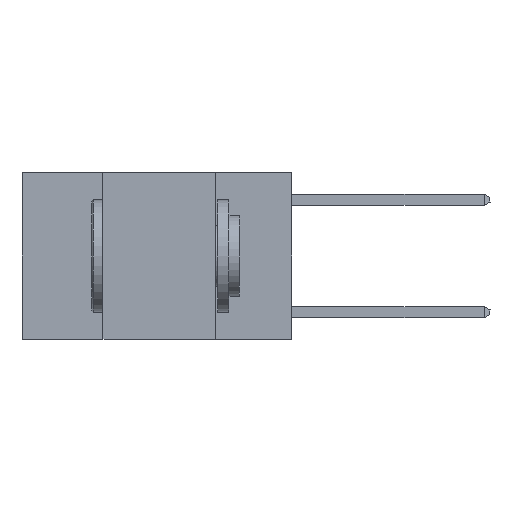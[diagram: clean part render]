
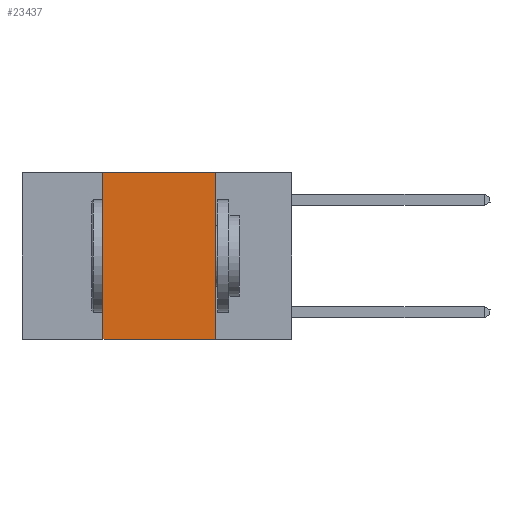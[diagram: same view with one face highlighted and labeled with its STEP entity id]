
A CAD part, left-side view. The second image highlights one B-rep face of the part: STEP entity #23437.
In plain terms, the highlighted planar face has unit normal (-1, 0, 0).
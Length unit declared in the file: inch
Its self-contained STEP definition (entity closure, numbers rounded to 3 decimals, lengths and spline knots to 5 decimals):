
#451 = EDGE_CURVE ( 'NONE', #24099, #14234, #26014, .T. ) ;
#692 = VECTOR ( 'NONE', #10924, 39.37008 ) ;
#1348 = CARTESIAN_POINT ( 'NONE',  ( 0., 0.42, 0. ) ) ;
#1947 = CARTESIAN_POINT ( 'NONE',  ( 0., 0.42, 0. ) ) ;
#2583 = VECTOR ( 'NONE', #11522, 39.37008 ) ;
#2958 = CARTESIAN_POINT ( 'NONE',  ( 0., 0.17, 0. ) ) ;
#5213 = EDGE_CURVE ( 'NONE', #24099, #6766, #21648, .T. ) ;
#5501 = EDGE_CURVE ( 'NONE', #16096, #6766, #16313, .T. ) ;
#5898 = EDGE_LOOP ( 'NONE', ( #19561, #11397, #6461, #11877 ) ) ;
#6102 = DIRECTION ( 'NONE',  ( 0., -1., 0. ) ) ;
#6274 = DIRECTION ( 'NONE',  ( 0., 0., 1. ) ) ;
#6461 = ORIENTED_EDGE ( 'NONE', *, *, #451, .F. ) ;
#6766 = VERTEX_POINT ( 'NONE', #22417 ) ;
#10639 = CARTESIAN_POINT ( 'NONE',  ( 0., 0.17, 0. ) ) ;
#10895 = CARTESIAN_POINT ( 'NONE',  ( 0., 0.6, -0.37 ) ) ;
#10924 = DIRECTION ( 'NONE',  ( 0., -1., 0. ) ) ;
#11397 = ORIENTED_EDGE ( 'NONE', *, *, #26266, .F. ) ;
#11522 = DIRECTION ( 'NONE',  ( 0., 0., -1. ) ) ;
#11877 = ORIENTED_EDGE ( 'NONE', *, *, #5213, .T. ) ;
#12086 = CARTESIAN_POINT ( 'NONE',  ( 0., 0.6, 0. ) ) ;
#12967 = CARTESIAN_POINT ( 'NONE',  ( 0., 0.6, 0. ) ) ;
#14234 = VERTEX_POINT ( 'NONE', #1947 ) ;
#16096 = VERTEX_POINT ( 'NONE', #10639 ) ;
#16313 = LINE ( 'NONE', #2958, #2583 ) ;
#18604 = DIRECTION ( 'NONE',  ( 1., 0., 0. ) ) ;
#19198 = LINE ( 'NONE', #12967, #692 ) ;
#19561 = ORIENTED_EDGE ( 'NONE', *, *, #5501, .F. ) ;
#19984 = CARTESIAN_POINT ( 'NONE',  ( 0., 0.42, -0.37 ) ) ;
#20130 = VECTOR ( 'NONE', #6274, 39.37008 ) ;
#21083 = FACE_OUTER_BOUND ( 'NONE', #5898, .T. ) ;
#21614 = VECTOR ( 'NONE', #6102, 39.37008 ) ;
#21648 = LINE ( 'NONE', #10895, #21614 ) ;
#22417 = CARTESIAN_POINT ( 'NONE',  ( 0., 0.17, -0.37 ) ) ;
#22470 = AXIS2_PLACEMENT_3D ( 'NONE', #12086, #18604, #27592 ) ;
#23437 = ADVANCED_FACE ( 'NONE', ( #21083 ), #25415, .F. ) ;
#24099 = VERTEX_POINT ( 'NONE', #19984 ) ;
#25415 = PLANE ( 'NONE',  #22470 ) ;
#26014 = LINE ( 'NONE', #1348, #20130 ) ;
#26266 = EDGE_CURVE ( 'NONE', #14234, #16096, #19198, .T. ) ;
#27592 = DIRECTION ( 'NONE',  ( 0., 0., -1. ) ) ;
